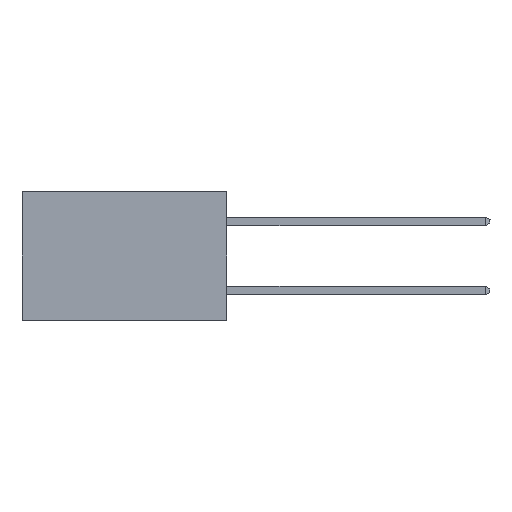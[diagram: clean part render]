
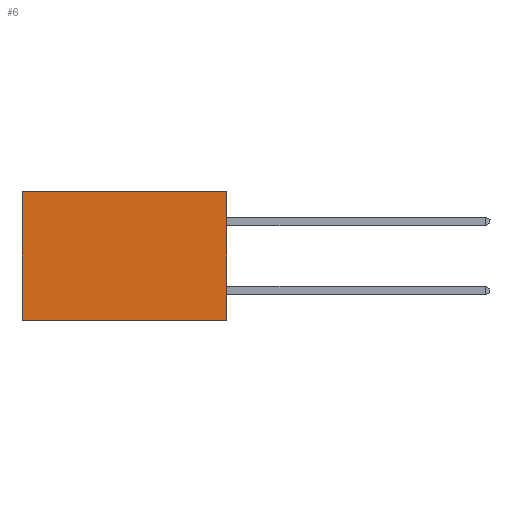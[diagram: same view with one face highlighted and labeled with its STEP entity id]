
A CAD part, left-side view. The second image highlights one B-rep face of the part: STEP entity #6.
In plain terms, the highlighted planar face has unit normal (-1, 0, 0).
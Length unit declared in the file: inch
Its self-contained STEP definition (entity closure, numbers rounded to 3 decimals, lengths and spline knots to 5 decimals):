
#6 = ADVANCED_FACE ( 'NONE', ( #6649 ), #1294, .F. ) ;
#1158 = VECTOR ( 'NONE', #6123, 39.37008 ) ;
#1294 = PLANE ( 'NONE',  #6827 ) ;
#1469 = LINE ( 'NONE', #4139, #8512 ) ;
#1605 = ORIENTED_EDGE ( 'NONE', *, *, #4399, .T. ) ;
#1615 = ORIENTED_EDGE ( 'NONE', *, *, #4348, .F. ) ;
#1634 = ORIENTED_EDGE ( 'NONE', *, *, #2529, .F. ) ;
#1652 = ORIENTED_EDGE ( 'NONE', *, *, #7600, .T. ) ;
#2529 = EDGE_CURVE ( 'NONE', #7063, #4639, #6701, .T. ) ;
#2796 = DIRECTION ( 'NONE',  ( 0., 0., -1. ) ) ;
#2923 = CARTESIAN_POINT ( 'NONE',  ( 0.277, 0.59, 0. ) ) ;
#3030 = EDGE_LOOP ( 'NONE', ( #1605, #1615, #1634, #1652 ) ) ;
#3702 = LINE ( 'NONE', #7548, #5338 ) ;
#3731 = CARTESIAN_POINT ( 'NONE',  ( 0.277, 0., 0. ) ) ;
#4139 = CARTESIAN_POINT ( 'NONE',  ( 0.277, 0.59, -0.37 ) ) ;
#4286 = VECTOR ( 'NONE', #7854, 39.37008 ) ;
#4348 = EDGE_CURVE ( 'NONE', #4639, #7467, #3702, .T. ) ;
#4399 = EDGE_CURVE ( 'NONE', #6248, #7467, #1469, .T. ) ;
#4639 = VERTEX_POINT ( 'NONE', #7945 ) ;
#5338 = VECTOR ( 'NONE', #5538, 39.37008 ) ;
#5538 = DIRECTION ( 'NONE',  ( 0., 1., 0. ) ) ;
#5644 = CARTESIAN_POINT ( 'NONE',  ( 0.277, 0., -0.37 ) ) ;
#5745 = CARTESIAN_POINT ( 'NONE',  ( 0.277, 0.59, -0.37 ) ) ;
#6123 = DIRECTION ( 'NONE',  ( 0., 0., -1. ) ) ;
#6248 = VERTEX_POINT ( 'NONE', #2923 ) ;
#6298 = DIRECTION ( 'NONE',  ( 1., 0., 0. ) ) ;
#6364 = DIRECTION ( 'NONE',  ( 0., 0., -1. ) ) ;
#6649 = FACE_OUTER_BOUND ( 'NONE', #3030, .T. ) ;
#6701 = LINE ( 'NONE', #5644, #1158 ) ;
#6827 = AXIS2_PLACEMENT_3D ( 'NONE', #8398, #6298, #6364 ) ;
#7063 = VERTEX_POINT ( 'NONE', #8089 ) ;
#7467 = VERTEX_POINT ( 'NONE', #5745 ) ;
#7548 = CARTESIAN_POINT ( 'NONE',  ( 0.277, 0., -0.37 ) ) ;
#7600 = EDGE_CURVE ( 'NONE', #7063, #6248, #7937, .T. ) ;
#7854 = DIRECTION ( 'NONE',  ( 0., 1., 0. ) ) ;
#7937 = LINE ( 'NONE', #3731, #4286 ) ;
#7945 = CARTESIAN_POINT ( 'NONE',  ( 0.277, 0., -0.37 ) ) ;
#8089 = CARTESIAN_POINT ( 'NONE',  ( 0.277, 0., 0. ) ) ;
#8398 = CARTESIAN_POINT ( 'NONE',  ( 0.277, 0., -0.37 ) ) ;
#8512 = VECTOR ( 'NONE', #2796, 39.37008 ) ;
